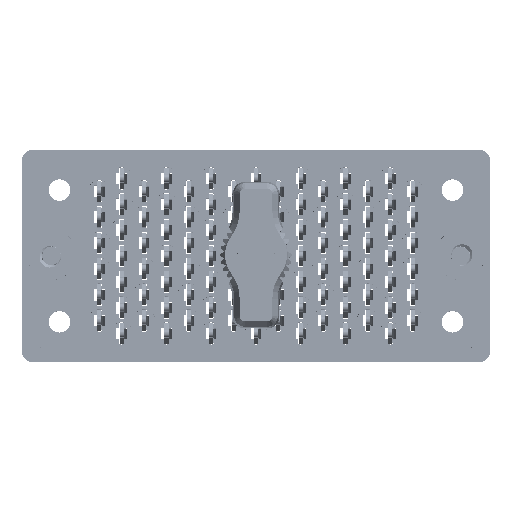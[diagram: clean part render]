
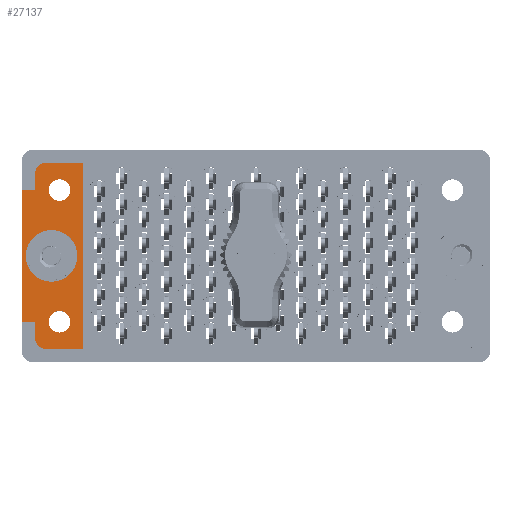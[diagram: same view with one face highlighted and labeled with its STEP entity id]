
A CAD part, top view. The second image highlights one B-rep face of the part: STEP entity #27137.
In plain terms, the highlighted planar face has unit normal (0, 0, 1).
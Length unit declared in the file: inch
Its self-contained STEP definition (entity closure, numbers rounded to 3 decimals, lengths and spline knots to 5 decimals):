
#770 = ORIENTED_EDGE ( 'NONE', *, *, #8511, .T. ) ;
#1193 = ORIENTED_EDGE ( 'NONE', *, *, #29418, .F. ) ;
#1268 = VECTOR ( 'NONE', #92009, 39.37008 ) ;
#1316 = DIRECTION ( 'NONE',  ( 0., 0., 1. ) ) ;
#2555 = EDGE_CURVE ( 'NONE', #56730, #44051, #78851, .T. ) ;
#3228 = DIRECTION ( 'NONE',  ( 0., 0., 1. ) ) ;
#4914 = DIRECTION ( 'NONE',  ( 1., 0., 0. ) ) ;
#5288 = FACE_OUTER_BOUND ( 'NONE', #42960, .T. ) ;
#5681 = AXIS2_PLACEMENT_3D ( 'NONE', #22614, #88840, #89782 ) ;
#5716 = LINE ( 'NONE', #23170, #15082 ) ;
#6451 = AXIS2_PLACEMENT_3D ( 'NONE', #86151, #40878, #63322 ) ;
#7451 = LINE ( 'NONE', #66873, #86796 ) ;
#7946 = ORIENTED_EDGE ( 'NONE', *, *, #2555, .F. ) ;
#8431 = CARTESIAN_POINT ( 'NONE',  ( -1.3375, 0., -0.117 ) ) ;
#8511 = EDGE_CURVE ( 'NONE', #42041, #52530, #63739, .T. ) ;
#8569 = DIRECTION ( 'NONE',  ( 0., 0., 1. ) ) ;
#10562 = CARTESIAN_POINT ( 'NONE',  ( -1.0785, 0.3825, -0.117 ) ) ;
#10723 = DIRECTION ( 'NONE',  ( 1., 0., 0. ) ) ;
#10812 = CARTESIAN_POINT ( 'NONE',  ( -1.2825, -0.478, -0.117 ) ) ;
#13435 = CARTESIAN_POINT ( 'NONE',  ( 0., -0.3825, -0.117 ) ) ;
#13455 = AXIS2_PLACEMENT_3D ( 'NONE', #49345, #48028, #78622 ) ;
#13891 = CARTESIAN_POINT ( 'NONE',  ( -1.2035, 0.3825, -0.117 ) ) ;
#14207 = VERTEX_POINT ( 'NONE', #87400 ) ;
#14869 = VECTOR ( 'NONE', #89676, 39.37008 ) ;
#15082 = VECTOR ( 'NONE', #32690, 39.37008 ) ;
#15777 = FACE_BOUND ( 'NONE', #66702, .T. ) ;
#16109 = DIRECTION ( 'NONE',  ( 1., 0., 0. ) ) ;
#17080 = LINE ( 'NONE', #78750, #35781 ) ;
#17378 = CARTESIAN_POINT ( 'NONE',  ( -1.005, 0.54, -0.117 ) ) ;
#20098 = EDGE_CURVE ( 'NONE', #93755, #42041, #17080, .T. ) ;
#21699 = CARTESIAN_POINT ( 'NONE',  ( -1.359, -0.3825, -0.117 ) ) ;
#21897 = CIRCLE ( 'NONE', #82499, 0.0625 ) ;
#22614 = CARTESIAN_POINT ( 'NONE',  ( -1.1875, 0., -0.117 ) ) ;
#23170 = CARTESIAN_POINT ( 'NONE',  ( -1.005, 0.617, -0.117 ) ) ;
#24819 = EDGE_LOOP ( 'NONE', ( #93427, #7946 ) ) ;
#24961 = CARTESIAN_POINT ( 'NONE',  ( -1.2205, 0.478, -0.117 ) ) ;
#26027 = EDGE_CURVE ( 'NONE', #44051, #56730, #21897, .T. ) ;
#27137 = ADVANCED_FACE ( 'NONE', ( #44976, #86955, #15777, #5288 ), #79582, .T. ) ;
#27265 = EDGE_CURVE ( 'NONE', #63227, #89062, #53092, .T. ) ;
#27696 = EDGE_CURVE ( 'NONE', #90483, #53265, #49588, .T. ) ;
#29046 = EDGE_CURVE ( 'NONE', #52530, #37652, #53935, .T. ) ;
#29418 = EDGE_CURVE ( 'NONE', #53265, #90483, #91130, .T. ) ;
#29707 = EDGE_CURVE ( 'NONE', #74205, #52132, #71392, .T. ) ;
#29977 = AXIS2_PLACEMENT_3D ( 'NONE', #82593, #8569, #16109 ) ;
#30378 = DIRECTION ( 'NONE',  ( 0., 0., 1. ) ) ;
#31134 = LINE ( 'NONE', #75286, #14869 ) ;
#31765 = CARTESIAN_POINT ( 'NONE',  ( -1.2205, 0.54, -0.117 ) ) ;
#32690 = DIRECTION ( 'NONE',  ( 0., 1., 0. ) ) ;
#33295 = VECTOR ( 'NONE', #94914, 39.37008 ) ;
#34409 = DIRECTION ( 'NONE',  ( 0., -1., 0. ) ) ;
#34961 = ORIENTED_EDGE ( 'NONE', *, *, #54077, .F. ) ;
#35781 = VECTOR ( 'NONE', #80413, 39.37008 ) ;
#37555 = EDGE_LOOP ( 'NONE', ( #1193, #94619 ) ) ;
#37652 = VERTEX_POINT ( 'NONE', #68061 ) ;
#38918 = CARTESIAN_POINT ( 'NONE',  ( -1.2205, -0.54, -0.117 ) ) ;
#39236 = ORIENTED_EDGE ( 'NONE', *, *, #87664, .T. ) ;
#40315 = ORIENTED_EDGE ( 'NONE', *, *, #29707, .F. ) ;
#40692 = EDGE_CURVE ( 'NONE', #44606, #51590, #82539, .T. ) ;
#40713 = EDGE_CURVE ( 'NONE', #63227, #44606, #31134, .T. ) ;
#40878 = DIRECTION ( 'NONE',  ( 0., 0., 1. ) ) ;
#40900 = CARTESIAN_POINT ( 'NONE',  ( -1.2825, 0., -0.117 ) ) ;
#42041 = VERTEX_POINT ( 'NONE', #31765 ) ;
#42960 = EDGE_LOOP ( 'NONE', ( #95927, #70525, #75015, #71323, #70947, #770, #43964, #49101, #39236, #53842 ) ) ;
#43455 = AXIS2_PLACEMENT_3D ( 'NONE', #52197, #30378, #96525 ) ;
#43964 = ORIENTED_EDGE ( 'NONE', *, *, #29046, .T. ) ;
#44051 = VERTEX_POINT ( 'NONE', #13891 ) ;
#44606 = VERTEX_POINT ( 'NONE', #10812 ) ;
#44976 = FACE_BOUND ( 'NONE', #37555, .T. ) ;
#46056 = CARTESIAN_POINT ( 'NONE',  ( -1.141, 0.3825, -0.117 ) ) ;
#46982 = DIRECTION ( 'NONE',  ( 0., -1., 0. ) ) ;
#48028 = DIRECTION ( 'NONE',  ( 0., 0., 1. ) ) ;
#48286 = VECTOR ( 'NONE', #61928, 39.37008 ) ;
#49101 = ORIENTED_EDGE ( 'NONE', *, *, #87551, .T. ) ;
#49345 = CARTESIAN_POINT ( 'NONE',  ( -1.141, -0.3825, -0.117 ) ) ;
#49588 = CIRCLE ( 'NONE', #57705, 0.0625 ) ;
#50849 = VERTEX_POINT ( 'NONE', #83621 ) ;
#51590 = VERTEX_POINT ( 'NONE', #38918 ) ;
#51596 = AXIS2_PLACEMENT_3D ( 'NONE', #60314, #1316, #90952 ) ;
#52132 = VERTEX_POINT ( 'NONE', #8431 ) ;
#52197 = CARTESIAN_POINT ( 'NONE',  ( -1.2205, -0.478, -0.117 ) ) ;
#52530 = VERTEX_POINT ( 'NONE', #52645 ) ;
#52645 = CARTESIAN_POINT ( 'NONE',  ( -1.2825, 0.478, -0.117 ) ) ;
#53092 = LINE ( 'NONE', #13435, #33295 ) ;
#53265 = VERTEX_POINT ( 'NONE', #60317 ) ;
#53842 = ORIENTED_EDGE ( 'NONE', *, *, #27265, .F. ) ;
#53935 = LINE ( 'NONE', #40900, #58607 ) ;
#54008 = DIRECTION ( 'NONE',  ( 0., 0., 1. ) ) ;
#54077 = EDGE_CURVE ( 'NONE', #52132, #74205, #56297, .T. ) ;
#55058 = CARTESIAN_POINT ( 'NONE',  ( -1.141, -0.3825, -0.117 ) ) ;
#55224 = CARTESIAN_POINT ( 'NONE',  ( -1.0785, -0.3825, -0.117 ) ) ;
#56297 = CIRCLE ( 'NONE', #5681, 0.15 ) ;
#56730 = VERTEX_POINT ( 'NONE', #10562 ) ;
#57705 = AXIS2_PLACEMENT_3D ( 'NONE', #55058, #3228, #10723 ) ;
#58607 = VECTOR ( 'NONE', #34409, 39.37008 ) ;
#60314 = CARTESIAN_POINT ( 'NONE',  ( -1.1875, 0., -0.117 ) ) ;
#60317 = CARTESIAN_POINT ( 'NONE',  ( -1.2035, -0.3825, -0.117 ) ) ;
#61928 = DIRECTION ( 'NONE',  ( -1., 0., 0. ) ) ;
#63227 = VERTEX_POINT ( 'NONE', #93544 ) ;
#63322 = DIRECTION ( 'NONE',  ( 1., 0., 0. ) ) ;
#63739 = CIRCLE ( 'NONE', #64643, 0.062 ) ;
#64643 = AXIS2_PLACEMENT_3D ( 'NONE', #24961, #54008, #83654 ) ;
#66702 = EDGE_LOOP ( 'NONE', ( #40315, #34961 ) ) ;
#66873 = CARTESIAN_POINT ( 'NONE',  ( -1.359, 0.617, -0.117 ) ) ;
#68061 = CARTESIAN_POINT ( 'NONE',  ( -1.2825, 0.3825, -0.117 ) ) ;
#69581 = CARTESIAN_POINT ( 'NONE',  ( 0., -0.54, -0.117 ) ) ;
#70132 = DIRECTION ( 'NONE',  ( 0., 0., 1. ) ) ;
#70525 = ORIENTED_EDGE ( 'NONE', *, *, #40692, .T. ) ;
#70947 = ORIENTED_EDGE ( 'NONE', *, *, #20098, .T. ) ;
#71323 = ORIENTED_EDGE ( 'NONE', *, *, #75302, .T. ) ;
#71392 = CIRCLE ( 'NONE', #51596, 0.15 ) ;
#72511 = LINE ( 'NONE', #69581, #1268 ) ;
#73665 = EDGE_CURVE ( 'NONE', #14207, #51590, #72511, .T. ) ;
#74205 = VERTEX_POINT ( 'NONE', #84285 ) ;
#74375 = CARTESIAN_POINT ( 'NONE',  ( 0., 0.3825, -0.117 ) ) ;
#75015 = ORIENTED_EDGE ( 'NONE', *, *, #73665, .F. ) ;
#75286 = CARTESIAN_POINT ( 'NONE',  ( -1.2825, 0., -0.117 ) ) ;
#75302 = EDGE_CURVE ( 'NONE', #14207, #93755, #5716, .T. ) ;
#78622 = DIRECTION ( 'NONE',  ( 1., 0., 0. ) ) ;
#78750 = CARTESIAN_POINT ( 'NONE',  ( 0., 0.54, -0.117 ) ) ;
#78851 = CIRCLE ( 'NONE', #29977, 0.0625 ) ;
#79582 = PLANE ( 'NONE',  #6451 ) ;
#80413 = DIRECTION ( 'NONE',  ( -1., 0., 0. ) ) ;
#82099 = LINE ( 'NONE', #74375, #48286 ) ;
#82499 = AXIS2_PLACEMENT_3D ( 'NONE', #46056, #70132, #4914 ) ;
#82539 = CIRCLE ( 'NONE', #43455, 0.062 ) ;
#82593 = CARTESIAN_POINT ( 'NONE',  ( -1.141, 0.3825, -0.117 ) ) ;
#83621 = CARTESIAN_POINT ( 'NONE',  ( -1.359, 0.3825, -0.117 ) ) ;
#83654 = DIRECTION ( 'NONE',  ( 1., 0., 0. ) ) ;
#84285 = CARTESIAN_POINT ( 'NONE',  ( -1.0375, 0., -0.117 ) ) ;
#86151 = CARTESIAN_POINT ( 'NONE',  ( -1.359, -0.617, -0.117 ) ) ;
#86796 = VECTOR ( 'NONE', #46982, 39.37008 ) ;
#86955 = FACE_BOUND ( 'NONE', #24819, .T. ) ;
#87400 = CARTESIAN_POINT ( 'NONE',  ( -1.005, -0.54, -0.117 ) ) ;
#87551 = EDGE_CURVE ( 'NONE', #37652, #50849, #82099, .T. ) ;
#87664 = EDGE_CURVE ( 'NONE', #50849, #89062, #7451, .T. ) ;
#88840 = DIRECTION ( 'NONE',  ( 0., 0., 1. ) ) ;
#89062 = VERTEX_POINT ( 'NONE', #21699 ) ;
#89676 = DIRECTION ( 'NONE',  ( 0., -1., 0. ) ) ;
#89782 = DIRECTION ( 'NONE',  ( 1., 0., 0. ) ) ;
#90483 = VERTEX_POINT ( 'NONE', #55224 ) ;
#90952 = DIRECTION ( 'NONE',  ( 1., 0., 0. ) ) ;
#91130 = CIRCLE ( 'NONE', #13455, 0.0625 ) ;
#92009 = DIRECTION ( 'NONE',  ( -1., 0., 0. ) ) ;
#93427 = ORIENTED_EDGE ( 'NONE', *, *, #26027, .F. ) ;
#93544 = CARTESIAN_POINT ( 'NONE',  ( -1.2825, -0.3825, -0.117 ) ) ;
#93755 = VERTEX_POINT ( 'NONE', #17378 ) ;
#94619 = ORIENTED_EDGE ( 'NONE', *, *, #27696, .F. ) ;
#94914 = DIRECTION ( 'NONE',  ( -1., 0., 0. ) ) ;
#95927 = ORIENTED_EDGE ( 'NONE', *, *, #40713, .T. ) ;
#96525 = DIRECTION ( 'NONE',  ( 1., 0., 0. ) ) ;
